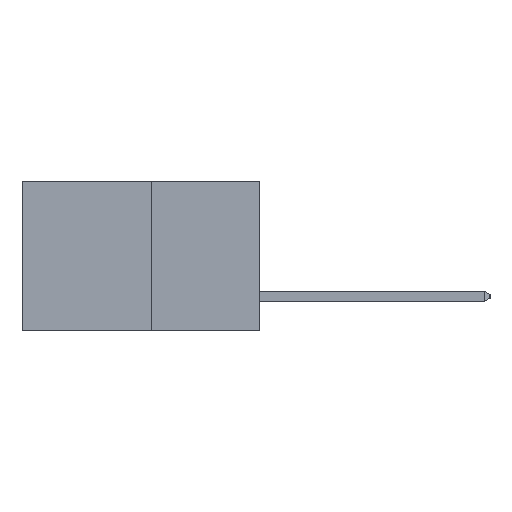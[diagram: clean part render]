
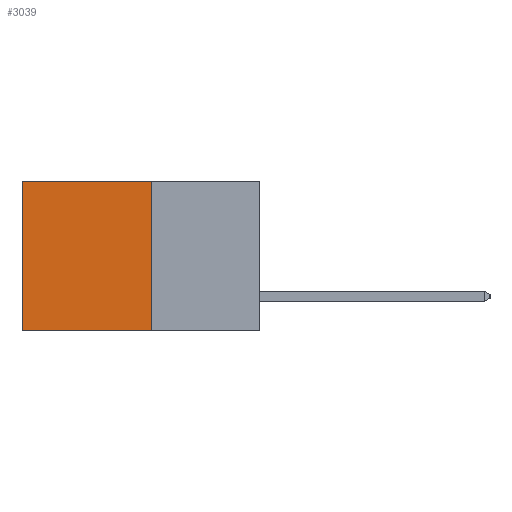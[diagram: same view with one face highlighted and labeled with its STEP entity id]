
A CAD part, left-side view. The second image highlights one B-rep face of the part: STEP entity #3039.
In plain terms, the highlighted planar face has unit normal (-1, 0, 0).
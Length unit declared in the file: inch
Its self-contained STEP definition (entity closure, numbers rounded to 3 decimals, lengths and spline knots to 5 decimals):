
#233 = CARTESIAN_POINT ( 'NONE',  ( 0.277, 0.59, -0.37 ) ) ;
#424 = EDGE_CURVE ( 'NONE', #7642, #1188, #12872, .T. ) ;
#1112 = CARTESIAN_POINT ( 'NONE',  ( 0.277, 0.27, -0.37 ) ) ;
#1188 = VERTEX_POINT ( 'NONE', #9612 ) ;
#1702 = CARTESIAN_POINT ( 'NONE',  ( 0.277, 0.27, -0.37 ) ) ;
#1795 = EDGE_CURVE ( 'NONE', #7454, #2010, #6918, .T. ) ;
#2010 = VERTEX_POINT ( 'NONE', #1702 ) ;
#2548 = EDGE_CURVE ( 'NONE', #2010, #1188, #12644, .T. ) ;
#3039 = ADVANCED_FACE ( 'NONE', ( #6115 ), #8261, .F. ) ;
#3335 = VECTOR ( 'NONE', #7124, 39.37008 ) ;
#3466 = VECTOR ( 'NONE', #4122, 39.37008 ) ;
#3678 = VECTOR ( 'NONE', #7713, 39.37008 ) ;
#3800 = ORIENTED_EDGE ( 'NONE', *, *, #14782, .T. ) ;
#4122 = DIRECTION ( 'NONE',  ( 0., 1., 0. ) ) ;
#4240 = CARTESIAN_POINT ( 'NONE',  ( 0.277, 0.27, 0. ) ) ;
#4789 = AXIS2_PLACEMENT_3D ( 'NONE', #1112, #7002, #12386 ) ;
#5447 = DIRECTION ( 'NONE',  ( 0., 1., 0. ) ) ;
#5925 = CARTESIAN_POINT ( 'NONE',  ( 0.277, 0.27, -0.37 ) ) ;
#6115 = FACE_OUTER_BOUND ( 'NONE', #10832, .T. ) ;
#6144 = CARTESIAN_POINT ( 'NONE',  ( 0.277, 0.59, 0. ) ) ;
#6274 = ORIENTED_EDGE ( 'NONE', *, *, #1795, .F. ) ;
#6918 = LINE ( 'NONE', #7479, #3678 ) ;
#7002 = DIRECTION ( 'NONE',  ( 1., 0., 0. ) ) ;
#7124 = DIRECTION ( 'NONE',  ( 0., 0., -1. ) ) ;
#7454 = VERTEX_POINT ( 'NONE', #8220 ) ;
#7479 = CARTESIAN_POINT ( 'NONE',  ( 0.277, 0.27, -0.37 ) ) ;
#7642 = VERTEX_POINT ( 'NONE', #6144 ) ;
#7713 = DIRECTION ( 'NONE',  ( 0., 0., -1. ) ) ;
#8220 = CARTESIAN_POINT ( 'NONE',  ( 0.277, 0.27, 0. ) ) ;
#8261 = PLANE ( 'NONE',  #4789 ) ;
#9612 = CARTESIAN_POINT ( 'NONE',  ( 0.277, 0.59, -0.37 ) ) ;
#10832 = EDGE_LOOP ( 'NONE', ( #14829, #15170, #6274, #3800 ) ) ;
#12084 = VECTOR ( 'NONE', #5447, 39.37008 ) ;
#12386 = DIRECTION ( 'NONE',  ( 0., 0., -1. ) ) ;
#12459 = LINE ( 'NONE', #4240, #12084 ) ;
#12644 = LINE ( 'NONE', #5925, #3466 ) ;
#12872 = LINE ( 'NONE', #233, #3335 ) ;
#14782 = EDGE_CURVE ( 'NONE', #7454, #7642, #12459, .T. ) ;
#14829 = ORIENTED_EDGE ( 'NONE', *, *, #424, .T. ) ;
#15170 = ORIENTED_EDGE ( 'NONE', *, *, #2548, .F. ) ;
